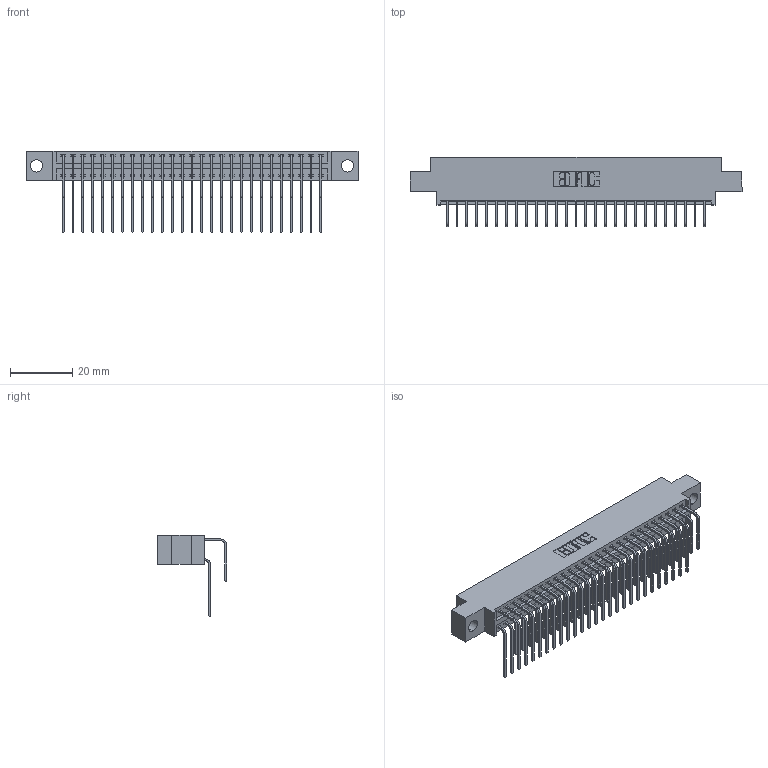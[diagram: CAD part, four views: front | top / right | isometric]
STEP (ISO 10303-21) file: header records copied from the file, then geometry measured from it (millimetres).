
FILE_DESCRIPTION (( 'STEP AP203' ), '1' );
FILE_NAME ('346-054-558-804.STEP', '2022-05-21T04:17:08', ( '' ), ( '' ), 'SwSTEP 2.0', 'SolidWorks 2020', '' );
FILE_SCHEMA (( 'CONFIG_CONTROL_DESIGN' ));
Length unit declared in the file: inch
Products named in the file (4): 346 Part_0.170 Offset - 0.156 Dia-TH; 345-292-001_558 Tail - 2; 345-292-001_558 559 Tail - 1; 346-054-558-804
Assembly tree (55 placements, depth 2):
  346-054-558-804
    346 Part_0.170 Offset - 0.156 Dia-TH
    345-292-001_558 559 Tail - 1  x27
    345-292-001_558 Tail - 2  x27
Bounding box: 106.3 x 22.16 x 26.16 mm (x, y, z)
Volume: 10299.9 mm3; surface area: 15444.1 mm2
Topology: 55 solids, 55 shells, 3056 faces, 9071 edges, 5974 vertices
Faces by surface type: plane 2092, cylinder 964
Entity records: 21975 total; most frequent: CARTESIAN_POINT 3701, ORIENTED_EDGE 3582, DIRECTION 3283, EDGE_CURVE 1791, LINE 1511, VECTOR 1511, VERTEX_POINT 1190, AXIS2_PLACEMENT_3D 886
